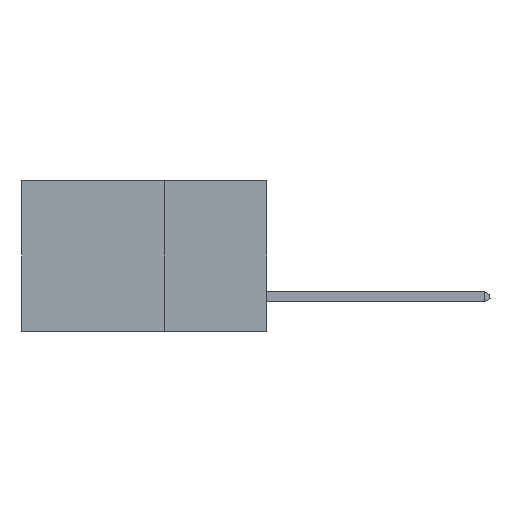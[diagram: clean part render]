
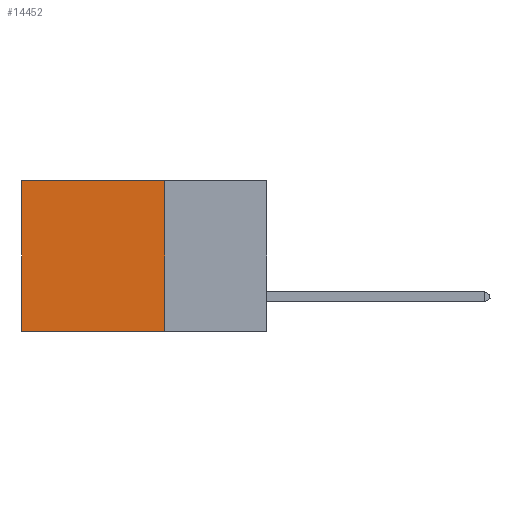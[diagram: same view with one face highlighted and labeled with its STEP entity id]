
A CAD part, left-side view. The second image highlights one B-rep face of the part: STEP entity #14452.
In plain terms, the highlighted planar face has unit normal (-1, 0, 0).
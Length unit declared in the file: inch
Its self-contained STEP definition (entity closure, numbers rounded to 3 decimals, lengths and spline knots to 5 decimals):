
#1650 = LINE ( 'NONE', #26362, #13177 ) ;
#5334 = DIRECTION ( 'NONE',  ( 0., 0., -1. ) ) ;
#5950 = CARTESIAN_POINT ( 'NONE',  ( 0.2875, 0.25, 0. ) ) ;
#7102 = LINE ( 'NONE', #19647, #41071 ) ;
#8898 = ORIENTED_EDGE ( 'NONE', *, *, #11416, .F. ) ;
#11416 = EDGE_CURVE ( 'NONE', #39663, #30968, #41736, .T. ) ;
#11881 = ORIENTED_EDGE ( 'NONE', *, *, #33839, .T. ) ;
#13177 = VECTOR ( 'NONE', #15489, 39.37008 ) ;
#14148 = CARTESIAN_POINT ( 'NONE',  ( 0.2875, 0.6, -0.37 ) ) ;
#14452 = ADVANCED_FACE ( 'NONE', ( #44811 ), #27958, .F. ) ;
#14889 = LINE ( 'NONE', #17618, #30872 ) ;
#15076 = EDGE_CURVE ( 'NONE', #30968, #35843, #14889, .T. ) ;
#15423 = CARTESIAN_POINT ( 'NONE',  ( 0.2875, 0.25, -0.37 ) ) ;
#15489 = DIRECTION ( 'NONE',  ( 0., 1., 0. ) ) ;
#17618 = CARTESIAN_POINT ( 'NONE',  ( 0.2875, 0.25, -0.37 ) ) ;
#18132 = CARTESIAN_POINT ( 'NONE',  ( 0.2875, 0.25, 0. ) ) ;
#19647 = CARTESIAN_POINT ( 'NONE',  ( 0.2875, 0.6, 0. ) ) ;
#21486 = AXIS2_PLACEMENT_3D ( 'NONE', #5950, #35388, #39148 ) ;
#21789 = DIRECTION ( 'NONE',  ( 0., 0., -1. ) ) ;
#26362 = CARTESIAN_POINT ( 'NONE',  ( 0.2875, 0.25, 0. ) ) ;
#26573 = ORIENTED_EDGE ( 'NONE', *, *, #28778, .T. ) ;
#26639 = ORIENTED_EDGE ( 'NONE', *, *, #15076, .F. ) ;
#27958 = PLANE ( 'NONE',  #21486 ) ;
#28191 = CARTESIAN_POINT ( 'NONE',  ( 0.2875, 0.6, 0. ) ) ;
#28778 = EDGE_CURVE ( 'NONE', #30417, #35843, #7102, .T. ) ;
#30417 = VERTEX_POINT ( 'NONE', #28191 ) ;
#30711 = VECTOR ( 'NONE', #21789, 39.37008 ) ;
#30872 = VECTOR ( 'NONE', #36749, 39.37008 ) ;
#30968 = VERTEX_POINT ( 'NONE', #15423 ) ;
#33839 = EDGE_CURVE ( 'NONE', #39663, #30417, #1650, .T. ) ;
#35388 = DIRECTION ( 'NONE',  ( 1., 0., 0. ) ) ;
#35552 = CARTESIAN_POINT ( 'NONE',  ( 0.2875, 0.25, 0. ) ) ;
#35843 = VERTEX_POINT ( 'NONE', #14148 ) ;
#36320 = EDGE_LOOP ( 'NONE', ( #26573, #26639, #8898, #11881 ) ) ;
#36749 = DIRECTION ( 'NONE',  ( 0., 1., 0. ) ) ;
#39148 = DIRECTION ( 'NONE',  ( 0., 0., -1. ) ) ;
#39663 = VERTEX_POINT ( 'NONE', #35552 ) ;
#41071 = VECTOR ( 'NONE', #5334, 39.37008 ) ;
#41736 = LINE ( 'NONE', #18132, #30711 ) ;
#44811 = FACE_OUTER_BOUND ( 'NONE', #36320, .T. ) ;
